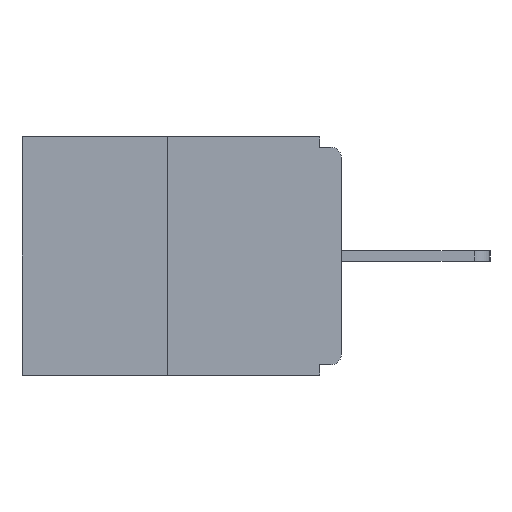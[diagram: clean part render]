
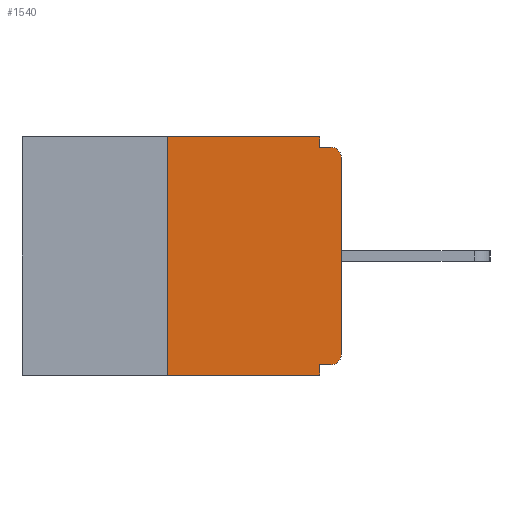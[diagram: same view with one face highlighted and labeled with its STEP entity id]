
A CAD part, left-side view. The second image highlights one B-rep face of the part: STEP entity #1540.
In plain terms, the highlighted planar face has unit normal (-1, 0, 0).
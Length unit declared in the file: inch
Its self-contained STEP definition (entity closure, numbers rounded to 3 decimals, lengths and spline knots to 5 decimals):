
#411 = DIRECTION ( 'NONE',  ( 0., 0., -1. ) ) ;
#796 = CARTESIAN_POINT ( 'NONE',  ( 0., 0.015, -0.03 ) ) ;
#840 = CARTESIAN_POINT ( 'NONE',  ( 0., 0.031, -0.328 ) ) ;
#890 = DIRECTION ( 'NONE',  ( 0., 0., 1. ) ) ;
#940 = LINE ( 'NONE', #13471, #10816 ) ;
#1540 = ADVANCED_FACE ( 'NONE', ( #4838 ), #5028, .F. ) ;
#1739 = VERTEX_POINT ( 'NONE', #20193 ) ;
#1975 = CARTESIAN_POINT ( 'NONE',  ( 0., 0.46, 0. ) ) ;
#2231 = ORIENTED_EDGE ( 'NONE', *, *, #9125, .T. ) ;
#2863 = EDGE_CURVE ( 'NONE', #6223, #3433, #3444, .T. ) ;
#3086 = VECTOR ( 'NONE', #17967, 39.37008 ) ;
#3170 = CARTESIAN_POINT ( 'NONE',  ( 0., 0.25, 0. ) ) ;
#3293 = VECTOR ( 'NONE', #15840, 39.37008 ) ;
#3433 = VERTEX_POINT ( 'NONE', #18262 ) ;
#3444 = LINE ( 'NONE', #16137, #3293 ) ;
#3456 = VERTEX_POINT ( 'NONE', #7087 ) ;
#3859 = LINE ( 'NONE', #6697, #17996 ) ;
#4120 = VECTOR ( 'NONE', #17541, 39.37008 ) ;
#4593 = ORIENTED_EDGE ( 'NONE', *, *, #15182, .T. ) ;
#4838 = FACE_OUTER_BOUND ( 'NONE', #10217, .T. ) ;
#4950 = AXIS2_PLACEMENT_3D ( 'NONE', #796, #10363, #5732 ) ;
#5028 = PLANE ( 'NONE',  #19043 ) ;
#5040 = CIRCLE ( 'NONE', #11302, 0.015 ) ;
#5478 = CARTESIAN_POINT ( 'NONE',  ( 0., 0.031, 0. ) ) ;
#5732 = DIRECTION ( 'NONE',  ( 0., 0., -1. ) ) ;
#5733 = ORIENTED_EDGE ( 'NONE', *, *, #8585, .F. ) ;
#6223 = VERTEX_POINT ( 'NONE', #3170 ) ;
#6697 = CARTESIAN_POINT ( 'NONE',  ( 0., 0.46, -0.343 ) ) ;
#6997 = LINE ( 'NONE', #13491, #16504 ) ;
#7087 = CARTESIAN_POINT ( 'NONE',  ( 0., 0.015, -0.328 ) ) ;
#7544 = ORIENTED_EDGE ( 'NONE', *, *, #12755, .F. ) ;
#7789 = EDGE_CURVE ( 'NONE', #18692, #10959, #8800, .T. ) ;
#7912 = VERTEX_POINT ( 'NONE', #11162 ) ;
#8227 = CIRCLE ( 'NONE', #4950, 0.015 ) ;
#8465 = ORIENTED_EDGE ( 'NONE', *, *, #2863, .F. ) ;
#8585 = EDGE_CURVE ( 'NONE', #19282, #6223, #940, .T. ) ;
#8662 = LINE ( 'NONE', #5478, #3086 ) ;
#8733 = ORIENTED_EDGE ( 'NONE', *, *, #7789, .F. ) ;
#8800 = LINE ( 'NONE', #13306, #15338 ) ;
#8899 = EDGE_CURVE ( 'NONE', #7912, #13279, #18101, .T. ) ;
#9043 = CARTESIAN_POINT ( 'NONE',  ( 0., 0.031, -0.015 ) ) ;
#9125 = EDGE_CURVE ( 'NONE', #19282, #10959, #3859, .T. ) ;
#10020 = DIRECTION ( 'NONE',  ( 0., -1., 0. ) ) ;
#10217 = EDGE_LOOP ( 'NONE', ( #8465, #5733, #2231, #8733, #12163, #4593, #18841, #12467, #17642, #7544 ) ) ;
#10363 = DIRECTION ( 'NONE',  ( -1., 0., 0. ) ) ;
#10640 = EDGE_CURVE ( 'NONE', #13279, #1739, #8227, .T. ) ;
#10816 = VECTOR ( 'NONE', #19689, 39.37008 ) ;
#10959 = VERTEX_POINT ( 'NONE', #19010 ) ;
#11132 = DIRECTION ( 'NONE',  ( 1., 0., 0. ) ) ;
#11162 = CARTESIAN_POINT ( 'NONE',  ( 0., 0., -0.313 ) ) ;
#11302 = AXIS2_PLACEMENT_3D ( 'NONE', #17657, #12978, #13175 ) ;
#12163 = ORIENTED_EDGE ( 'NONE', *, *, #17925, .F. ) ;
#12467 = ORIENTED_EDGE ( 'NONE', *, *, #10640, .T. ) ;
#12755 = EDGE_CURVE ( 'NONE', #3433, #17469, #8662, .T. ) ;
#12821 = CARTESIAN_POINT ( 'NONE',  ( 0., 0.25, -0.343 ) ) ;
#12978 = DIRECTION ( 'NONE',  ( -1., 0., 0. ) ) ;
#13171 = LINE ( 'NONE', #19388, #4120 ) ;
#13175 = DIRECTION ( 'NONE',  ( 0., 0., -1. ) ) ;
#13279 = VERTEX_POINT ( 'NONE', #18531 ) ;
#13306 = CARTESIAN_POINT ( 'NONE',  ( 0., 0.031, -0.343 ) ) ;
#13471 = CARTESIAN_POINT ( 'NONE',  ( 0., 0.25, 0. ) ) ;
#13491 = CARTESIAN_POINT ( 'NONE',  ( 0., 0., -0.015 ) ) ;
#15022 = DIRECTION ( 'NONE',  ( 0., 0., -1. ) ) ;
#15182 = EDGE_CURVE ( 'NONE', #3456, #7912, #5040, .T. ) ;
#15227 = EDGE_CURVE ( 'NONE', #17469, #1739, #6997, .T. ) ;
#15338 = VECTOR ( 'NONE', #15022, 39.37008 ) ;
#15840 = DIRECTION ( 'NONE',  ( 0., -1., 0. ) ) ;
#16137 = CARTESIAN_POINT ( 'NONE',  ( 0., 0.46, 0. ) ) ;
#16342 = VECTOR ( 'NONE', #890, 39.37008 ) ;
#16504 = VECTOR ( 'NONE', #17042, 39.37008 ) ;
#17042 = DIRECTION ( 'NONE',  ( 0., -1., 0. ) ) ;
#17469 = VERTEX_POINT ( 'NONE', #9043 ) ;
#17541 = DIRECTION ( 'NONE',  ( 0., 1., 0. ) ) ;
#17642 = ORIENTED_EDGE ( 'NONE', *, *, #15227, .F. ) ;
#17657 = CARTESIAN_POINT ( 'NONE',  ( 0., 0.015, -0.313 ) ) ;
#17925 = EDGE_CURVE ( 'NONE', #3456, #18692, #13171, .T. ) ;
#17967 = DIRECTION ( 'NONE',  ( 0., 0., -1. ) ) ;
#17996 = VECTOR ( 'NONE', #10020, 39.37008 ) ;
#18101 = LINE ( 'NONE', #19954, #16342 ) ;
#18262 = CARTESIAN_POINT ( 'NONE',  ( 0., 0.031, 0. ) ) ;
#18531 = CARTESIAN_POINT ( 'NONE',  ( 0., 0., -0.03 ) ) ;
#18692 = VERTEX_POINT ( 'NONE', #840 ) ;
#18841 = ORIENTED_EDGE ( 'NONE', *, *, #8899, .T. ) ;
#19010 = CARTESIAN_POINT ( 'NONE',  ( 0., 0.031, -0.343 ) ) ;
#19043 = AXIS2_PLACEMENT_3D ( 'NONE', #1975, #11132, #411 ) ;
#19282 = VERTEX_POINT ( 'NONE', #12821 ) ;
#19388 = CARTESIAN_POINT ( 'NONE',  ( 0., 0., -0.328 ) ) ;
#19689 = DIRECTION ( 'NONE',  ( 0., 0., 1. ) ) ;
#19954 = CARTESIAN_POINT ( 'NONE',  ( 0., 0., 0. ) ) ;
#20193 = CARTESIAN_POINT ( 'NONE',  ( 0., 0.015, -0.015 ) ) ;
